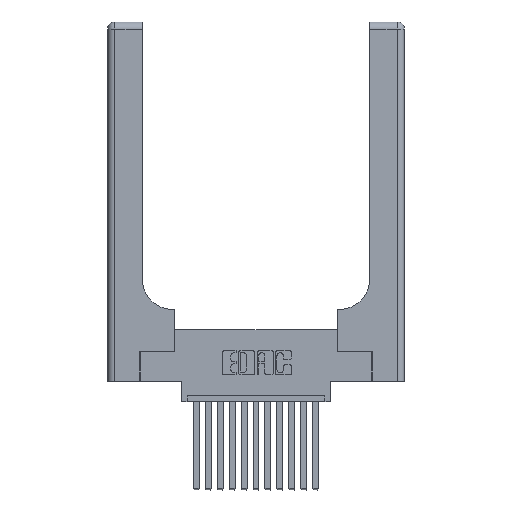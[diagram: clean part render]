
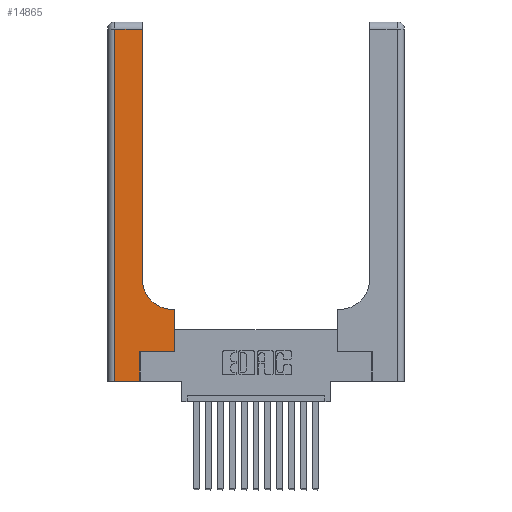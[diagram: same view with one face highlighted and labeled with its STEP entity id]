
A CAD part, top view. The second image highlights one B-rep face of the part: STEP entity #14865.
In plain terms, the highlighted planar face has unit normal (0, 0, 1).
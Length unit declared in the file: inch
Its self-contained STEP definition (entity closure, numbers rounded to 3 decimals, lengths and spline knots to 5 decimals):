
#68 = EDGE_CURVE ( 'NONE', #13767, #5232, #12471, .T. ) ;
#110 = ORIENTED_EDGE ( 'NONE', *, *, #68, .T. ) ;
#117 = CARTESIAN_POINT ( 'NONE',  ( 0.5585, 0.25, 0.37 ) ) ;
#126 = VECTOR ( 'NONE', #6244, 39.37008 ) ;
#139 = ORIENTED_EDGE ( 'NONE', *, *, #8735, .T. ) ;
#344 = CARTESIAN_POINT ( 'NONE',  ( 0., 3., 0.37 ) ) ;
#666 = CARTESIAN_POINT ( 'NONE',  ( 0., 0., 0.37 ) ) ;
#1107 = FACE_OUTER_BOUND ( 'NONE', #3724, .T. ) ;
#1217 = VECTOR ( 'NONE', #6357, 39.37008 ) ;
#1316 = EDGE_CURVE ( 'NONE', #10995, #12120, #11823, .T. ) ;
#1345 = CARTESIAN_POINT ( 'NONE',  ( 0.06, 3., 0.37 ) ) ;
#1449 = CARTESIAN_POINT ( 'NONE',  ( 0.06, 2.94, 0.37 ) ) ;
#2017 = AXIS2_PLACEMENT_3D ( 'NONE', #11455, #7379, #14266 ) ;
#2451 = CARTESIAN_POINT ( 'NONE',  ( 0.2915, 3., 0.37 ) ) ;
#2605 = EDGE_CURVE ( 'NONE', #15049, #13767, #5805, .T. ) ;
#3241 = DIRECTION ( 'NONE',  ( -1., 0., 0. ) ) ;
#3246 = ORIENTED_EDGE ( 'NONE', *, *, #17197, .T. ) ;
#3611 = LINE ( 'NONE', #666, #4872 ) ;
#3724 = EDGE_LOOP ( 'NONE', ( #139, #5832, #4641, #3246, #12409, #13035, #6698, #8851, #110 ) ) ;
#4483 = EDGE_CURVE ( 'NONE', #12120, #6298, #7042, .T. ) ;
#4641 = ORIENTED_EDGE ( 'NONE', *, *, #4483, .T. ) ;
#4683 = DIRECTION ( 'NONE',  ( 0., 1., 0. ) ) ;
#4872 = VECTOR ( 'NONE', #10169, 39.37008 ) ;
#5232 = VERTEX_POINT ( 'NONE', #7522 ) ;
#5558 = CARTESIAN_POINT ( 'NONE',  ( 0.5415, 0.6, 0.37 ) ) ;
#5805 = LINE ( 'NONE', #6145, #7511 ) ;
#5832 = ORIENTED_EDGE ( 'NONE', *, *, #1316, .T. ) ;
#6145 = CARTESIAN_POINT ( 'NONE',  ( 0.2915, 0.6, 0.37 ) ) ;
#6243 = VERTEX_POINT ( 'NONE', #16147 ) ;
#6244 = DIRECTION ( 'NONE',  ( -1., 0., 0. ) ) ;
#6298 = VERTEX_POINT ( 'NONE', #15034 ) ;
#6357 = DIRECTION ( 'NONE',  ( 0., 1., 0. ) ) ;
#6698 = ORIENTED_EDGE ( 'NONE', *, *, #15756, .T. ) ;
#6990 = DIRECTION ( 'NONE',  ( 1., 0., 0. ) ) ;
#7042 = LINE ( 'NONE', #1345, #15965 ) ;
#7379 = DIRECTION ( 'NONE',  ( 0., 0., -1. ) ) ;
#7417 = LINE ( 'NONE', #2451, #1217 ) ;
#7511 = VECTOR ( 'NONE', #15683, 39.37008 ) ;
#7522 = CARTESIAN_POINT ( 'NONE',  ( 0.2915, 0.85, 0.37 ) ) ;
#8105 = DIRECTION ( 'NONE',  ( 0., 1., 0. ) ) ;
#8735 = EDGE_CURVE ( 'NONE', #5232, #10995, #7417, .T. ) ;
#8851 = ORIENTED_EDGE ( 'NONE', *, *, #2605, .T. ) ;
#8996 = VECTOR ( 'NONE', #8105, 39.37008 ) ;
#9371 = VERTEX_POINT ( 'NONE', #117 ) ;
#9897 = CARTESIAN_POINT ( 'NONE',  ( 0.269, 0., 0.37 ) ) ;
#9967 = DIRECTION ( 'NONE',  ( 0., 0., -1. ) ) ;
#10169 = DIRECTION ( 'NONE',  ( 1., 0., 0. ) ) ;
#10300 = CARTESIAN_POINT ( 'NONE',  ( 0.5585, 0.6, 0.37 ) ) ;
#10837 = AXIS2_PLACEMENT_3D ( 'NONE', #344, #9967, #3241 ) ;
#10876 = DIRECTION ( 'NONE',  ( 0., -1., 0. ) ) ;
#10995 = VERTEX_POINT ( 'NONE', #17107 ) ;
#11342 = EDGE_CURVE ( 'NONE', #15199, #6243, #12234, .T. ) ;
#11455 = CARTESIAN_POINT ( 'NONE',  ( 0.5415, 0.85, 0.37 ) ) ;
#11579 = LINE ( 'NONE', #14761, #8996 ) ;
#11602 = VECTOR ( 'NONE', #6990, 39.37008 ) ;
#11646 = EDGE_CURVE ( 'NONE', #6243, #9371, #13961, .T. ) ;
#11823 = LINE ( 'NONE', #17135, #126 ) ;
#12120 = VERTEX_POINT ( 'NONE', #1449 ) ;
#12234 = LINE ( 'NONE', #9897, #17298 ) ;
#12409 = ORIENTED_EDGE ( 'NONE', *, *, #11342, .T. ) ;
#12471 = CIRCLE ( 'NONE', #2017, 0.25 ) ;
#13035 = ORIENTED_EDGE ( 'NONE', *, *, #11646, .T. ) ;
#13767 = VERTEX_POINT ( 'NONE', #5558 ) ;
#13961 = LINE ( 'NONE', #13983, #11602 ) ;
#13983 = CARTESIAN_POINT ( 'NONE',  ( 0.269, 0.25, 0.37 ) ) ;
#14266 = DIRECTION ( 'NONE',  ( 1., 0., 0. ) ) ;
#14761 = CARTESIAN_POINT ( 'NONE',  ( 0.5585, 0.25, 0.37 ) ) ;
#14865 = ADVANCED_FACE ( 'NONE', ( #1107 ), #16608, .F. ) ;
#15034 = CARTESIAN_POINT ( 'NONE',  ( 0.06, 0., 0.37 ) ) ;
#15049 = VERTEX_POINT ( 'NONE', #10300 ) ;
#15199 = VERTEX_POINT ( 'NONE', #16211 ) ;
#15683 = DIRECTION ( 'NONE',  ( -1., 0., 0. ) ) ;
#15756 = EDGE_CURVE ( 'NONE', #9371, #15049, #11579, .T. ) ;
#15965 = VECTOR ( 'NONE', #10876, 39.37008 ) ;
#16147 = CARTESIAN_POINT ( 'NONE',  ( 0.269, 0.25, 0.37 ) ) ;
#16211 = CARTESIAN_POINT ( 'NONE',  ( 0.269, 0., 0.37 ) ) ;
#16608 = PLANE ( 'NONE',  #10837 ) ;
#17107 = CARTESIAN_POINT ( 'NONE',  ( 0.2915, 2.94, 0.37 ) ) ;
#17135 = CARTESIAN_POINT ( 'NONE',  ( 0., 2.94, 0.37 ) ) ;
#17197 = EDGE_CURVE ( 'NONE', #6298, #15199, #3611, .T. ) ;
#17298 = VECTOR ( 'NONE', #4683, 39.37008 ) ;
